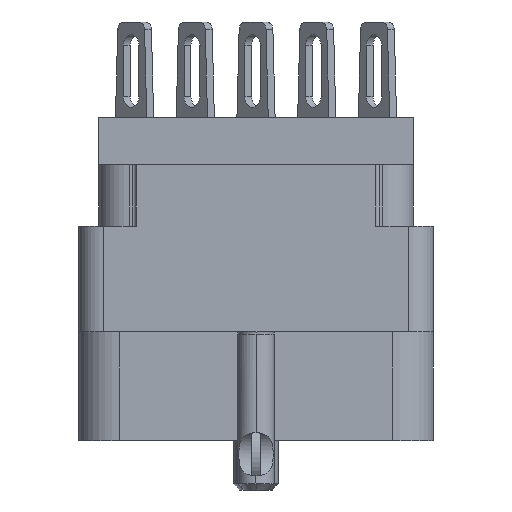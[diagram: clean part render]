
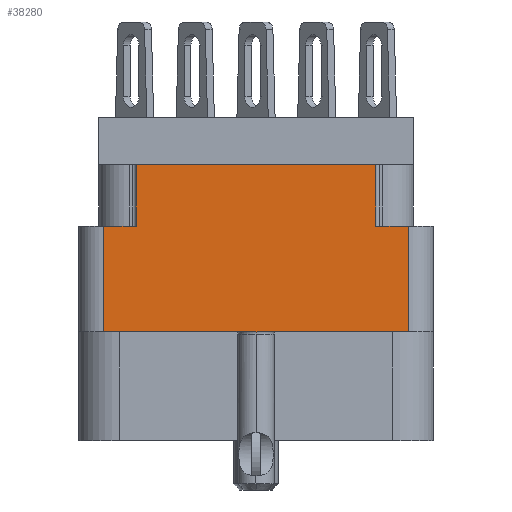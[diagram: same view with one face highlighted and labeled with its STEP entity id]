
A CAD part, left-side view. The second image highlights one B-rep face of the part: STEP entity #38280.
In plain terms, the highlighted planar face has unit normal (-1, 0, 0).
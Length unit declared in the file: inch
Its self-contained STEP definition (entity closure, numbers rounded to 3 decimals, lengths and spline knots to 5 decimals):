
#1725 = DIRECTION ( 'NONE',  ( -1., 0., 0. ) ) ;
#2063 = DIRECTION ( 'NONE',  ( 0., -1., 0. ) ) ;
#2166 = DIRECTION ( 'NONE',  ( 0., 0., 1. ) ) ;
#2377 = ORIENTED_EDGE ( 'NONE', *, *, #38415, .T. ) ;
#2996 = LINE ( 'NONE', #33474, #20733 ) ;
#4048 = LINE ( 'NONE', #4906, #30647 ) ;
#4510 = ORIENTED_EDGE ( 'NONE', *, *, #4960, .T. ) ;
#4610 = CARTESIAN_POINT ( 'NONE',  ( -1., 0.296, -0.117 ) ) ;
#4906 = CARTESIAN_POINT ( 'NONE',  ( -1., 0.438, -0.268 ) ) ;
#4960 = EDGE_CURVE ( 'NONE', #7847, #16074, #17920, .T. ) ;
#5182 = EDGE_CURVE ( 'NONE', #8851, #44909, #4048, .T. ) ;
#5544 = VERTEX_POINT ( 'NONE', #25525 ) ;
#7847 = VERTEX_POINT ( 'NONE', #19035 ) ;
#7980 = CARTESIAN_POINT ( 'NONE',  ( -1., 0.376, -0.798 ) ) ;
#8185 = VERTEX_POINT ( 'NONE', #13717 ) ;
#8271 = VERTEX_POINT ( 'NONE', #32004 ) ;
#8851 = VERTEX_POINT ( 'NONE', #43237 ) ;
#9046 = VECTOR ( 'NONE', #42576, 39.37008 ) ;
#10356 = ORIENTED_EDGE ( 'NONE', *, *, #5182, .F. ) ;
#11218 = LINE ( 'NONE', #7980, #21225 ) ;
#11949 = FACE_OUTER_BOUND ( 'NONE', #38743, .T. ) ;
#12775 = AXIS2_PLACEMENT_3D ( 'NONE', #22780, #1725, #29888 ) ;
#13717 = CARTESIAN_POINT ( 'NONE',  ( -1., -0.296, -0.117 ) ) ;
#13999 = LINE ( 'NONE', #17592, #9046 ) ;
#14246 = VECTOR ( 'NONE', #17587, 39.37008 ) ;
#16074 = VERTEX_POINT ( 'NONE', #19541 ) ;
#16104 = CARTESIAN_POINT ( 'NONE',  ( -1., 0.296, -0.268 ) ) ;
#17587 = DIRECTION ( 'NONE',  ( 0., 0., 1. ) ) ;
#17592 = CARTESIAN_POINT ( 'NONE',  ( -1., -0.296, -0.268 ) ) ;
#17920 = LINE ( 'NONE', #31711, #35103 ) ;
#19035 = CARTESIAN_POINT ( 'NONE',  ( -1., 0.376, -0.529 ) ) ;
#19541 = CARTESIAN_POINT ( 'NONE',  ( -1., -0.376, -0.529 ) ) ;
#19821 = DIRECTION ( 'NONE',  ( 0., 0., 1. ) ) ;
#19855 = CARTESIAN_POINT ( 'NONE',  ( -1., 0.438, -0.117 ) ) ;
#20733 = VECTOR ( 'NONE', #2166, 39.37008 ) ;
#21225 = VECTOR ( 'NONE', #36317, 39.37008 ) ;
#22780 = CARTESIAN_POINT ( 'NONE',  ( -1., -0.376, -0.798 ) ) ;
#25525 = CARTESIAN_POINT ( 'NONE',  ( -1., -0.296, -0.268 ) ) ;
#25676 = VERTEX_POINT ( 'NONE', #4610 ) ;
#27219 = EDGE_CURVE ( 'NONE', #25676, #8185, #35231, .T. ) ;
#27718 = CARTESIAN_POINT ( 'NONE',  ( -1., 0.296, -0.268 ) ) ;
#28780 = EDGE_CURVE ( 'NONE', #5544, #8271, #13999, .T. ) ;
#29281 = ORIENTED_EDGE ( 'NONE', *, *, #36866, .F. ) ;
#29547 = ORIENTED_EDGE ( 'NONE', *, *, #27219, .F. ) ;
#29888 = DIRECTION ( 'NONE',  ( 0., 0., 1. ) ) ;
#29960 = DIRECTION ( 'NONE',  ( 0., -1., 0. ) ) ;
#30647 = VECTOR ( 'NONE', #29960, 39.37008 ) ;
#31711 = CARTESIAN_POINT ( 'NONE',  ( -1., 0., -0.529 ) ) ;
#32004 = CARTESIAN_POINT ( 'NONE',  ( -1., -0.376, -0.268 ) ) ;
#32450 = EDGE_CURVE ( 'NONE', #16074, #8271, #2996, .T. ) ;
#33255 = EDGE_CURVE ( 'NONE', #7847, #8851, #11218, .T. ) ;
#33474 = CARTESIAN_POINT ( 'NONE',  ( -1., -0.376, -0.798 ) ) ;
#33587 = VECTOR ( 'NONE', #2063, 39.37008 ) ;
#33786 = CARTESIAN_POINT ( 'NONE',  ( -1., -0.296, -0.268 ) ) ;
#35103 = VECTOR ( 'NONE', #42575, 39.37008 ) ;
#35231 = LINE ( 'NONE', #19855, #33587 ) ;
#36317 = DIRECTION ( 'NONE',  ( 0., 0., 1. ) ) ;
#36528 = ORIENTED_EDGE ( 'NONE', *, *, #28780, .F. ) ;
#36866 = EDGE_CURVE ( 'NONE', #44909, #25676, #37592, .T. ) ;
#37452 = LINE ( 'NONE', #33786, #44629 ) ;
#37592 = LINE ( 'NONE', #27718, #14246 ) ;
#38280 = ADVANCED_FACE ( 'NONE', ( #11949 ), #40027, .T. ) ;
#38415 = EDGE_CURVE ( 'NONE', #5544, #8185, #37452, .T. ) ;
#38743 = EDGE_LOOP ( 'NONE', ( #42215, #4510, #45600, #36528, #2377, #29547, #29281, #10356 ) ) ;
#40027 = PLANE ( 'NONE',  #12775 ) ;
#42215 = ORIENTED_EDGE ( 'NONE', *, *, #33255, .F. ) ;
#42575 = DIRECTION ( 'NONE',  ( 0., -1., 0. ) ) ;
#42576 = DIRECTION ( 'NONE',  ( 0., -1., 0. ) ) ;
#43237 = CARTESIAN_POINT ( 'NONE',  ( -1., 0.376, -0.268 ) ) ;
#44629 = VECTOR ( 'NONE', #19821, 39.37008 ) ;
#44909 = VERTEX_POINT ( 'NONE', #16104 ) ;
#45600 = ORIENTED_EDGE ( 'NONE', *, *, #32450, .T. ) ;
